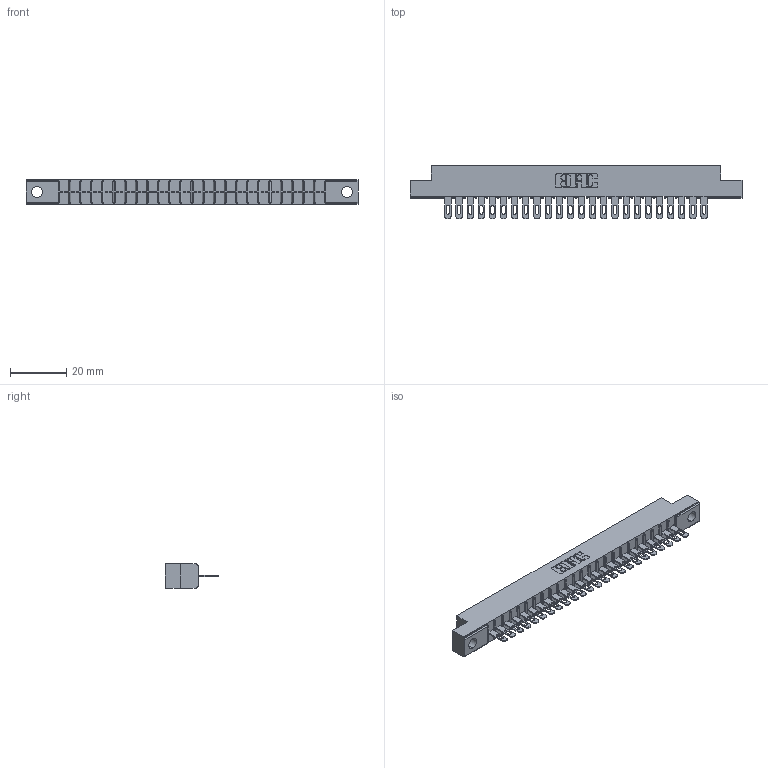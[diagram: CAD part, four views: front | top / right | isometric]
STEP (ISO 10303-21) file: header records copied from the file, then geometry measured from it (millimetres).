
FILE_DESCRIPTION (( 'STEP AP203' ), '1' );
FILE_NAME ('316-024-400-104.STEP', '2020-09-22T21:17:38', ( '' ), ( '' ), 'SwSTEP 2.0', 'SolidWorks 2020', '' );
FILE_SCHEMA (( 'CONFIG_CONTROL_DESIGN' ));
Length unit declared in the file: inch
Products named in the file (3): 306-290-001_100; 316-024-400-104; 306 Part_.156 Dia
Assembly tree (25 placements, depth 2):
  316-024-400-104
    306 Part_.156 Dia
    306-290-001_100  x24
Bounding box: 118.11 x 18.87 x 8.71 mm (x, y, z)
Volume: 8061.8 mm3; surface area: 12218 mm2
Topology: 25 solids, 25 shells, 1954 faces, 5512 edges, 3544 vertices
Faces by surface type: plane 1282, cylinder 576, sphere 96
Entity records: 25295 total; most frequent: CARTESIAN_POINT 4249, ORIENTED_EDGE 4208, DIRECTION 4184, EDGE_CURVE 2104, VECTOR 1642, LINE 1642, VERTEX_POINT 1336, AXIS2_PLACEMENT_3D 1271
